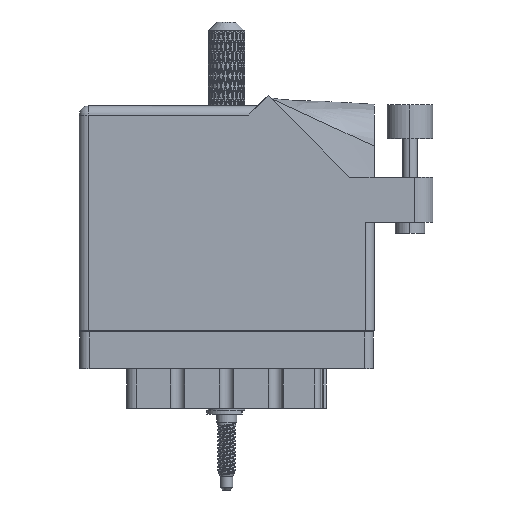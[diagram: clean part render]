
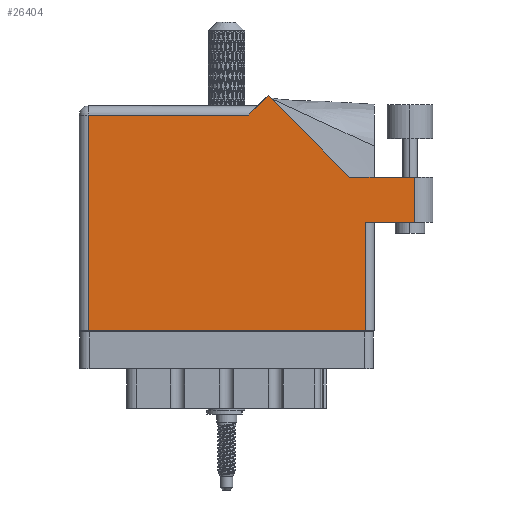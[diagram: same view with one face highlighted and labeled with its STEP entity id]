
A CAD part, front view. The second image highlights one B-rep face of the part: STEP entity #26404.
In plain terms, the highlighted face is planar.
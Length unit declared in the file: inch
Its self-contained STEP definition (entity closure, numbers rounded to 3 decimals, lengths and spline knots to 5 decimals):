
#129 = VECTOR ( 'NONE', #17944, 39.37008 ) ;
#325 = CARTESIAN_POINT ( 'NONE',  ( 0.062, 0., 0. ) ) ;
#546 = ORIENTED_EDGE ( 'NONE', *, *, #82247, .T. ) ;
#1643 = LINE ( 'NONE', #44294, #80596 ) ;
#1711 = CARTESIAN_POINT ( 'NONE',  ( 2.285, 1.044, 0. ) ) ;
#2403 = LINE ( 'NONE', #59291, #90463 ) ;
#2530 = ORIENTED_EDGE ( 'NONE', *, *, #7112, .T. ) ;
#2557 = CARTESIAN_POINT ( 'NONE',  ( 1.948, 0., 0. ) ) ;
#3213 = VERTEX_POINT ( 'NONE', #24042 ) ;
#5647 = VECTOR ( 'NONE', #58460, 39.37008 ) ;
#6482 = CARTESIAN_POINT ( 'NONE',  ( 1.217, 1.53, 0. ) ) ;
#7112 = EDGE_CURVE ( 'NONE', #15371, #49222, #106541, .T. ) ;
#9184 = EDGE_CURVE ( 'NONE', #42083, #37734, #1643, .T. ) ;
#9888 = CARTESIAN_POINT ( 'NONE',  ( 1.28771, 1.60071, 0. ) ) ;
#11676 = CARTESIAN_POINT ( 'NONE',  ( 0.062, 1.468, 0. ) ) ;
#14844 = ORIENTED_EDGE ( 'NONE', *, *, #40086, .T. ) ;
#15371 = VERTEX_POINT ( 'NONE', #11676 ) ;
#15534 = ORIENTED_EDGE ( 'NONE', *, *, #80053, .T. ) ;
#15552 = DIRECTION ( 'NONE',  ( -0.707, -0.707, 0. ) ) ;
#16629 = LINE ( 'NONE', #6482, #96800 ) ;
#17944 = DIRECTION ( 'NONE',  ( -1., 0., 0. ) ) ;
#18006 = DIRECTION ( 'NONE',  ( 0., 1., 0. ) ) ;
#21114 = ORIENTED_EDGE ( 'NONE', *, *, #83525, .T. ) ;
#22699 = VERTEX_POINT ( 'NONE', #2557 ) ;
#22936 = LINE ( 'NONE', #1711, #32030 ) ;
#24042 = CARTESIAN_POINT ( 'NONE',  ( 1.84442, 1.044, 0. ) ) ;
#26404 = ADVANCED_FACE ( 'NONE', ( #39135 ), #85176, .F. ) ;
#26440 = DIRECTION ( 'NONE',  ( -1., 0., 0. ) ) ;
#27759 = LINE ( 'NONE', #29873, #92420 ) ;
#28771 = CARTESIAN_POINT ( 'NONE',  ( 0.062, 0., 0. ) ) ;
#29873 = CARTESIAN_POINT ( 'NONE',  ( 0., 0., 0. ) ) ;
#30127 = VECTOR ( 'NONE', #33735, 39.37008 ) ;
#32030 = VECTOR ( 'NONE', #18006, 39.37008 ) ;
#33735 = DIRECTION ( 'NONE',  ( 0., 1., 0. ) ) ;
#34792 = CARTESIAN_POINT ( 'NONE',  ( 1.948, 0.737, 0. ) ) ;
#35633 = DIRECTION ( 'NONE',  ( -0.707, 0.707, 0. ) ) ;
#37734 = VERTEX_POINT ( 'NONE', #39567 ) ;
#37831 = DIRECTION ( 'NONE',  ( 1., 0., 0. ) ) ;
#39135 = FACE_OUTER_BOUND ( 'NONE', #60463, .T. ) ;
#39511 = CARTESIAN_POINT ( 'NONE',  ( 1.948, 0.737, 0. ) ) ;
#39567 = CARTESIAN_POINT ( 'NONE',  ( 2.285, 0.737, 0. ) ) ;
#40086 = EDGE_CURVE ( 'NONE', #56410, #3213, #2403, .T. ) ;
#42083 = VERTEX_POINT ( 'NONE', #39511 ) ;
#44294 = CARTESIAN_POINT ( 'NONE',  ( 2.01, 0.737, 0. ) ) ;
#45706 = VERTEX_POINT ( 'NONE', #9888 ) ;
#49222 = VERTEX_POINT ( 'NONE', #28771 ) ;
#49418 = CARTESIAN_POINT ( 'NONE',  ( 1.155, 1.468, 0. ) ) ;
#56410 = VERTEX_POINT ( 'NONE', #66744 ) ;
#58460 = DIRECTION ( 'NONE',  ( 0., -1., 0. ) ) ;
#59291 = CARTESIAN_POINT ( 'NONE',  ( 2.41, 1.044, 0. ) ) ;
#59807 = CARTESIAN_POINT ( 'NONE',  ( 0., 1.468, 0. ) ) ;
#60463 = EDGE_LOOP ( 'NONE', ( #93874, #21114, #14844, #60673, #546, #15534, #2530, #104776, #104727 ) ) ;
#60673 = ORIENTED_EDGE ( 'NONE', *, *, #63803, .T. ) ;
#63803 = EDGE_CURVE ( 'NONE', #3213, #45706, #82478, .T. ) ;
#66744 = CARTESIAN_POINT ( 'NONE',  ( 2.285, 1.044, 0. ) ) ;
#68118 = DIRECTION ( 'NONE',  ( -1., 0., 0. ) ) ;
#73682 = EDGE_CURVE ( 'NONE', #49222, #22699, #27759, .T. ) ;
#76967 = EDGE_CURVE ( 'NONE', #22699, #42083, #96061, .T. ) ;
#79873 = VECTOR ( 'NONE', #35633, 39.37008 ) ;
#80053 = EDGE_CURVE ( 'NONE', #88491, #15371, #89406, .T. ) ;
#80596 = VECTOR ( 'NONE', #95312, 39.37008 ) ;
#82247 = EDGE_CURVE ( 'NONE', #45706, #88491, #16629, .T. ) ;
#82478 = LINE ( 'NONE', #84800, #79873 ) ;
#83525 = EDGE_CURVE ( 'NONE', #37734, #56410, #22936, .T. ) ;
#84105 = CARTESIAN_POINT ( 'NONE',  ( 0., 1.53, 0. ) ) ;
#84800 = CARTESIAN_POINT ( 'NONE',  ( 1.84442, 1.044, 0. ) ) ;
#85176 = PLANE ( 'NONE',  #90163 ) ;
#88491 = VERTEX_POINT ( 'NONE', #49418 ) ;
#89406 = LINE ( 'NONE', #59807, #129 ) ;
#90163 = AXIS2_PLACEMENT_3D ( 'NONE', #84105, #101013, #68118 ) ;
#90463 = VECTOR ( 'NONE', #26440, 39.37008 ) ;
#92420 = VECTOR ( 'NONE', #37831, 39.37008 ) ;
#93874 = ORIENTED_EDGE ( 'NONE', *, *, #9184, .T. ) ;
#95312 = DIRECTION ( 'NONE',  ( 1., 0., 0. ) ) ;
#96061 = LINE ( 'NONE', #34792, #30127 ) ;
#96800 = VECTOR ( 'NONE', #15552, 39.37008 ) ;
#101013 = DIRECTION ( 'NONE',  ( 0., 0., -1. ) ) ;
#104727 = ORIENTED_EDGE ( 'NONE', *, *, #76967, .T. ) ;
#104776 = ORIENTED_EDGE ( 'NONE', *, *, #73682, .T. ) ;
#106541 = LINE ( 'NONE', #325, #5647 ) ;
